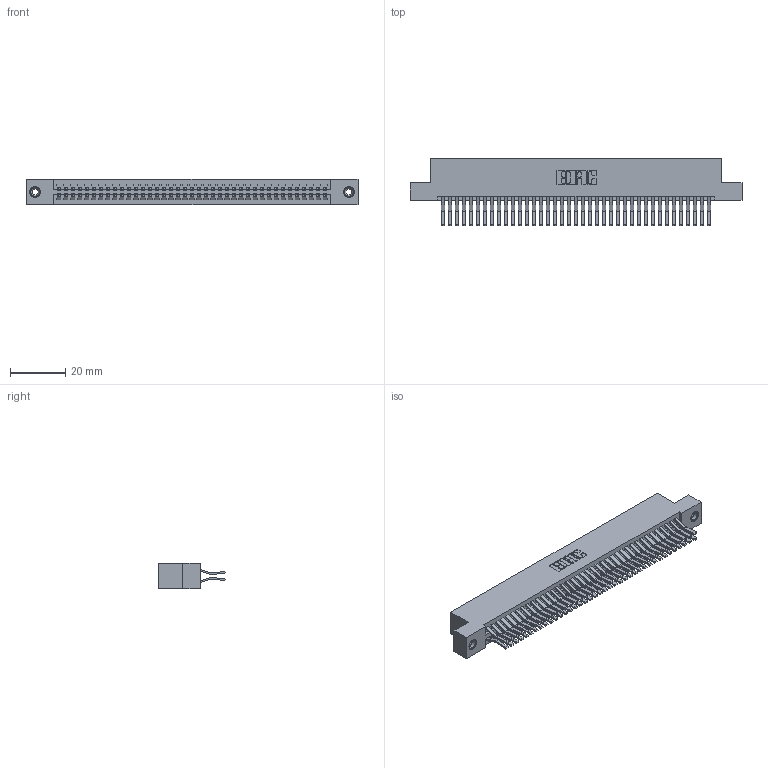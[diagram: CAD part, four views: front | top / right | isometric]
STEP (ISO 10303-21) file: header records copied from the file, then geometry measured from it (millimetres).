
FILE_DESCRIPTION (( 'STEP AP203' ), '1' );
FILE_NAME ('395-078-560-208.STEP', '2018-11-28T02:24:45', ( '' ), ( '' ), 'SwSTEP 2.0', 'SolidWorks 2016', '' );
FILE_SCHEMA (( 'CONFIG_CONTROL_DESIGN' ));
Length unit declared in the file: inch
Products named in the file (4): 395-078-560-208; 345 Part_Flush Mounting Lugs - 0.156 Dia-TI; 345-250-001_345-250-003-102; 345-292-001_560 Tail
Assembly tree (81 placements, depth 2):
  395-078-560-208
    345 Part_Flush Mounting Lugs - 0.156 Dia-TI
    345-292-001_560 Tail  x78
    345-250-001_345-250-003-102  x2
Bounding box: 120.27 x 24.45 x 9.4 mm (x, y, z)
Volume: 12160 mm3; surface area: 19244.7 mm2
Topology: 81 solids, 81 shells, 4242 faces, 12567 edges, 8266 vertices
Faces by surface type: plane 2686, cylinder 1540, cone 12, torus 4
Entity records: 32278 total; most frequent: CARTESIAN_POINT 5395, ORIENTED_EDGE 5322, DIRECTION 4791, EDGE_CURVE 2661, LINE 2349, VECTOR 2349, VERTEX_POINT 1768, AXIS2_PLACEMENT_3D 1221
